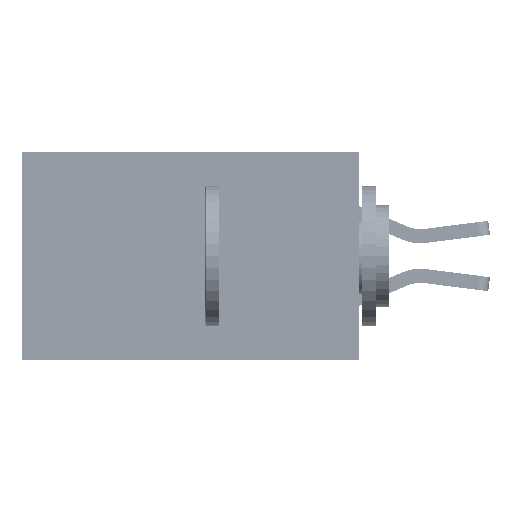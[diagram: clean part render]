
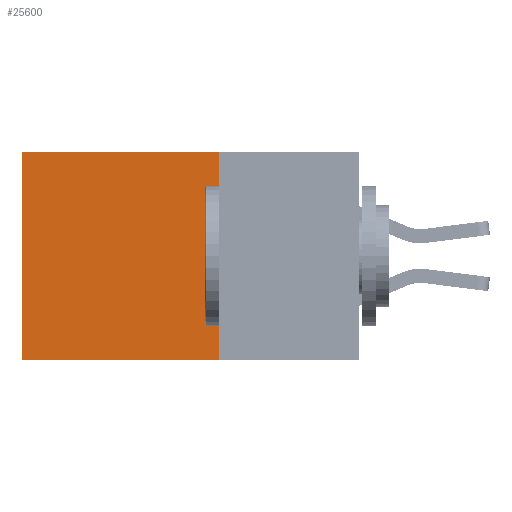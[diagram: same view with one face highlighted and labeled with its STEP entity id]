
A CAD part, left-side view. The second image highlights one B-rep face of the part: STEP entity #25600.
In plain terms, the highlighted planar face has unit normal (-1, 0, 0).
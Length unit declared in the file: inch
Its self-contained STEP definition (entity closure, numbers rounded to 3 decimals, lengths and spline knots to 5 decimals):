
#1299 = FACE_OUTER_BOUND ( 'NONE', #13922, .T. ) ;
#2535 = CARTESIAN_POINT ( 'NONE',  ( 0.2875, 0.25, -0.37 ) ) ;
#3285 = DIRECTION ( 'NONE',  ( 0., 1., 0. ) ) ;
#5286 = LINE ( 'NONE', #16796, #12830 ) ;
#6593 = VECTOR ( 'NONE', #3285, 39.37008 ) ;
#6743 = PLANE ( 'NONE',  #18903 ) ;
#8551 = VERTEX_POINT ( 'NONE', #2535 ) ;
#10115 = CARTESIAN_POINT ( 'NONE',  ( 0.2875, 0.6, -0.37 ) ) ;
#10253 = CARTESIAN_POINT ( 'NONE',  ( 0.2875, 0.25, -0.37 ) ) ;
#10458 = DIRECTION ( 'NONE',  ( 0., 0., -1. ) ) ;
#10583 = VERTEX_POINT ( 'NONE', #13110 ) ;
#10744 = EDGE_CURVE ( 'NONE', #8551, #10799, #24009, .T. ) ;
#10799 = VERTEX_POINT ( 'NONE', #10115 ) ;
#12830 = VECTOR ( 'NONE', #10458, 39.37008 ) ;
#13110 = CARTESIAN_POINT ( 'NONE',  ( 0.2875, 0.6, 0. ) ) ;
#13922 = EDGE_LOOP ( 'NONE', ( #30729, #28137, #16006, #28499 ) ) ;
#14036 = CARTESIAN_POINT ( 'NONE',  ( 0.2875, 0.25, 0. ) ) ;
#16006 = ORIENTED_EDGE ( 'NONE', *, *, #26321, .F. ) ;
#16796 = CARTESIAN_POINT ( 'NONE',  ( 0.2875, 0.25, 0. ) ) ;
#18903 = AXIS2_PLACEMENT_3D ( 'NONE', #26462, #32533, #35763 ) ;
#20590 = VECTOR ( 'NONE', #24925, 39.37008 ) ;
#23112 = LINE ( 'NONE', #37441, #20590 ) ;
#24009 = LINE ( 'NONE', #10253, #25539 ) ;
#24165 = EDGE_CURVE ( 'NONE', #10583, #10799, #23112, .T. ) ;
#24925 = DIRECTION ( 'NONE',  ( 0., 0., -1. ) ) ;
#25539 = VECTOR ( 'NONE', #32709, 39.37008 ) ;
#25600 = ADVANCED_FACE ( 'NONE', ( #1299 ), #6743, .F. ) ;
#25743 = VERTEX_POINT ( 'NONE', #14036 ) ;
#26321 = EDGE_CURVE ( 'NONE', #25743, #8551, #5286, .T. ) ;
#26462 = CARTESIAN_POINT ( 'NONE',  ( 0.2875, 0.25, 0. ) ) ;
#28137 = ORIENTED_EDGE ( 'NONE', *, *, #10744, .F. ) ;
#28499 = ORIENTED_EDGE ( 'NONE', *, *, #38649, .T. ) ;
#30729 = ORIENTED_EDGE ( 'NONE', *, *, #24165, .T. ) ;
#32319 = CARTESIAN_POINT ( 'NONE',  ( 0.2875, 0.25, 0. ) ) ;
#32533 = DIRECTION ( 'NONE',  ( 1., 0., 0. ) ) ;
#32709 = DIRECTION ( 'NONE',  ( 0., 1., 0. ) ) ;
#35763 = DIRECTION ( 'NONE',  ( 0., 0., -1. ) ) ;
#37441 = CARTESIAN_POINT ( 'NONE',  ( 0.2875, 0.6, 0. ) ) ;
#38649 = EDGE_CURVE ( 'NONE', #25743, #10583, #39304, .T. ) ;
#39304 = LINE ( 'NONE', #32319, #6593 ) ;
